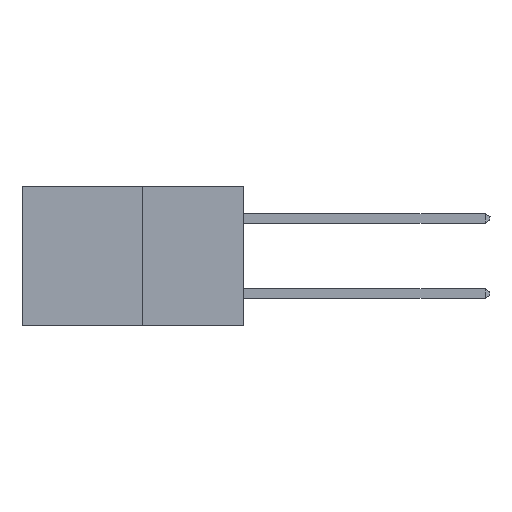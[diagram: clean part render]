
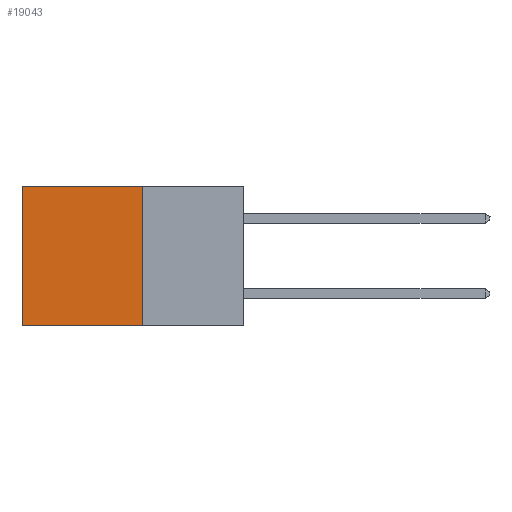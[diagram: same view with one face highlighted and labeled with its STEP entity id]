
A CAD part, left-side view. The second image highlights one B-rep face of the part: STEP entity #19043.
In plain terms, the highlighted planar face has unit normal (-1, 0, 0).
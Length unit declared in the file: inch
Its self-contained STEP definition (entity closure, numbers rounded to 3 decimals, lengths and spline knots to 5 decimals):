
#724 = DIRECTION ( 'NONE',  ( 1., 0., 0. ) ) ;
#767 = DIRECTION ( 'NONE',  ( 0., 1., 0. ) ) ;
#936 = CARTESIAN_POINT ( 'NONE',  ( 0.277, 0.27, 0. ) ) ;
#1213 = DIRECTION ( 'NONE',  ( 0., 1., 0. ) ) ;
#1531 = AXIS2_PLACEMENT_3D ( 'NONE', #14773, #724, #10982 ) ;
#2147 = EDGE_CURVE ( 'NONE', #15181, #8554, #19738, .T. ) ;
#3081 = VECTOR ( 'NONE', #767, 39.37008 ) ;
#3145 = EDGE_CURVE ( 'NONE', #15181, #13875, #8375, .T. ) ;
#3471 = EDGE_CURVE ( 'NONE', #8554, #17173, #19681, .T. ) ;
#3841 = ORIENTED_EDGE ( 'NONE', *, *, #3471, .T. ) ;
#5546 = CARTESIAN_POINT ( 'NONE',  ( 0.277, 0.59, -0.37 ) ) ;
#7549 = DIRECTION ( 'NONE',  ( 0., 0., -1. ) ) ;
#7616 = CARTESIAN_POINT ( 'NONE',  ( 0.277, 0.27, -0.37 ) ) ;
#8375 = LINE ( 'NONE', #7616, #16220 ) ;
#8554 = VERTEX_POINT ( 'NONE', #10307 ) ;
#9506 = DIRECTION ( 'NONE',  ( 0., 0., -1. ) ) ;
#9687 = CARTESIAN_POINT ( 'NONE',  ( 0.277, 0.59, -0.37 ) ) ;
#10307 = CARTESIAN_POINT ( 'NONE',  ( 0.277, 0.59, 0. ) ) ;
#10982 = DIRECTION ( 'NONE',  ( 0., 0., -1. ) ) ;
#11265 = FACE_OUTER_BOUND ( 'NONE', #16886, .T. ) ;
#12137 = VECTOR ( 'NONE', #1213, 39.37008 ) ;
#13875 = VERTEX_POINT ( 'NONE', #15185 ) ;
#14379 = PLANE ( 'NONE',  #1531 ) ;
#14773 = CARTESIAN_POINT ( 'NONE',  ( 0.277, 0.27, -0.37 ) ) ;
#15132 = CARTESIAN_POINT ( 'NONE',  ( 0.277, 0.27, -0.37 ) ) ;
#15181 = VERTEX_POINT ( 'NONE', #15852 ) ;
#15185 = CARTESIAN_POINT ( 'NONE',  ( 0.277, 0.27, -0.37 ) ) ;
#15503 = EDGE_CURVE ( 'NONE', #13875, #17173, #16315, .T. ) ;
#15852 = CARTESIAN_POINT ( 'NONE',  ( 0.277, 0.27, 0. ) ) ;
#16220 = VECTOR ( 'NONE', #7549, 39.37008 ) ;
#16315 = LINE ( 'NONE', #15132, #12137 ) ;
#16886 = EDGE_LOOP ( 'NONE', ( #3841, #19789, #18723, #20212 ) ) ;
#17173 = VERTEX_POINT ( 'NONE', #5546 ) ;
#18723 = ORIENTED_EDGE ( 'NONE', *, *, #3145, .F. ) ;
#19043 = ADVANCED_FACE ( 'NONE', ( #11265 ), #14379, .F. ) ;
#19164 = VECTOR ( 'NONE', #9506, 39.37008 ) ;
#19681 = LINE ( 'NONE', #9687, #19164 ) ;
#19738 = LINE ( 'NONE', #936, #3081 ) ;
#19789 = ORIENTED_EDGE ( 'NONE', *, *, #15503, .F. ) ;
#20212 = ORIENTED_EDGE ( 'NONE', *, *, #2147, .T. ) ;
